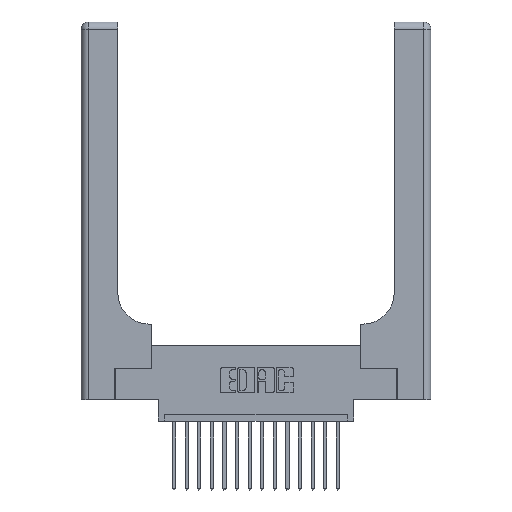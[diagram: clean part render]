
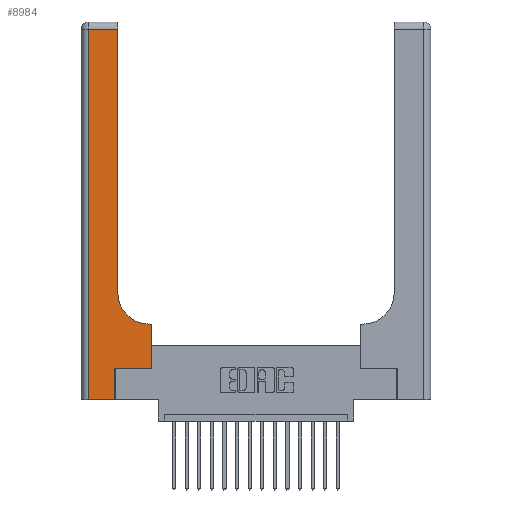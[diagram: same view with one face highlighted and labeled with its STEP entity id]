
A CAD part, top view. The second image highlights one B-rep face of the part: STEP entity #8984.
In plain terms, the highlighted planar face has unit normal (0, 0, 1).
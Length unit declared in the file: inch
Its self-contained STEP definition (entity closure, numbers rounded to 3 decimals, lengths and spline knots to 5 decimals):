
#375 = DIRECTION ( 'NONE',  ( 1., 0., 0. ) ) ;
#637 = ORIENTED_EDGE ( 'NONE', *, *, #4105, .T. ) ;
#830 = VECTOR ( 'NONE', #7267, 39.37008 ) ;
#835 = VERTEX_POINT ( 'NONE', #8999 ) ;
#1026 = CARTESIAN_POINT ( 'NONE',  ( 0.269, 0., 0.37 ) ) ;
#1332 = VERTEX_POINT ( 'NONE', #9746 ) ;
#1426 = LINE ( 'NONE', #15340, #8727 ) ;
#1843 = EDGE_CURVE ( 'NONE', #1332, #18634, #16734, .T. ) ;
#2083 = ORIENTED_EDGE ( 'NONE', *, *, #11551, .T. ) ;
#2517 = VECTOR ( 'NONE', #18983, 39.37008 ) ;
#3129 = DIRECTION ( 'NONE',  ( -1., 0., 0. ) ) ;
#3688 = LINE ( 'NONE', #12869, #2517 ) ;
#4105 = EDGE_CURVE ( 'NONE', #4329, #1332, #11870, .T. ) ;
#4235 = AXIS2_PLACEMENT_3D ( 'NONE', #13280, #10344, #4338 ) ;
#4329 = VERTEX_POINT ( 'NONE', #12420 ) ;
#4338 = DIRECTION ( 'NONE',  ( -1., 0., 0. ) ) ;
#4738 = DIRECTION ( 'NONE',  ( 1., 0., 0. ) ) ;
#4770 = CARTESIAN_POINT ( 'NONE',  ( 0., 2.94, 0.37 ) ) ;
#4840 = CARTESIAN_POINT ( 'NONE',  ( 0.06, 2.94, 0.37 ) ) ;
#6037 = AXIS2_PLACEMENT_3D ( 'NONE', #10881, #18533, #375 ) ;
#6086 = ORIENTED_EDGE ( 'NONE', *, *, #12809, .T. ) ;
#6097 = EDGE_CURVE ( 'NONE', #14502, #4329, #3688, .T. ) ;
#6288 = DIRECTION ( 'NONE',  ( 0., 1., 0. ) ) ;
#6469 = EDGE_LOOP ( 'NONE', ( #2083, #17138, #8055, #637, #8844, #6630, #14395, #15891, #6086 ) ) ;
#6630 = ORIENTED_EDGE ( 'NONE', *, *, #7451, .T. ) ;
#7267 = DIRECTION ( 'NONE',  ( -1., 0., 0. ) ) ;
#7451 = EDGE_CURVE ( 'NONE', #18634, #835, #7834, .T. ) ;
#7834 = LINE ( 'NONE', #14635, #14310 ) ;
#8055 = ORIENTED_EDGE ( 'NONE', *, *, #6097, .T. ) ;
#8470 = CARTESIAN_POINT ( 'NONE',  ( 0.5585, 0.6, 0.37 ) ) ;
#8727 = VECTOR ( 'NONE', #10784, 39.37008 ) ;
#8844 = ORIENTED_EDGE ( 'NONE', *, *, #1843, .T. ) ;
#8984 = ADVANCED_FACE ( 'NONE', ( #17605 ), #11674, .F. ) ;
#8999 = CARTESIAN_POINT ( 'NONE',  ( 0.5585, 0.25, 0.37 ) ) ;
#9328 = LINE ( 'NONE', #11988, #830 ) ;
#9746 = CARTESIAN_POINT ( 'NONE',  ( 0.269, 0., 0.37 ) ) ;
#9819 = EDGE_CURVE ( 'NONE', #835, #11036, #1426, .T. ) ;
#10344 = DIRECTION ( 'NONE',  ( 0., 0., -1. ) ) ;
#10585 = LINE ( 'NONE', #15235, #12728 ) ;
#10784 = DIRECTION ( 'NONE',  ( 0., 1., 0. ) ) ;
#10881 = CARTESIAN_POINT ( 'NONE',  ( 0.5415, 0.85, 0.37 ) ) ;
#11036 = VERTEX_POINT ( 'NONE', #8470 ) ;
#11212 = VERTEX_POINT ( 'NONE', #19307 ) ;
#11500 = CARTESIAN_POINT ( 'NONE',  ( 0.5415, 0.6, 0.37 ) ) ;
#11551 = EDGE_CURVE ( 'NONE', #11212, #17501, #10585, .T. ) ;
#11674 = PLANE ( 'NONE',  #4235 ) ;
#11870 = LINE ( 'NONE', #18333, #14059 ) ;
#11951 = VECTOR ( 'NONE', #19250, 39.37008 ) ;
#11988 = CARTESIAN_POINT ( 'NONE',  ( 0.2915, 0.6, 0.37 ) ) ;
#12420 = CARTESIAN_POINT ( 'NONE',  ( 0.06, 0., 0.37 ) ) ;
#12583 = EDGE_CURVE ( 'NONE', #11036, #14872, #9328, .T. ) ;
#12661 = LINE ( 'NONE', #4770, #15073 ) ;
#12728 = VECTOR ( 'NONE', #6288, 39.37008 ) ;
#12809 = EDGE_CURVE ( 'NONE', #14872, #11212, #14867, .T. ) ;
#12869 = CARTESIAN_POINT ( 'NONE',  ( 0.06, 3., 0.37 ) ) ;
#13280 = CARTESIAN_POINT ( 'NONE',  ( 0., 3., 0.37 ) ) ;
#14059 = VECTOR ( 'NONE', #4738, 39.37008 ) ;
#14068 = CARTESIAN_POINT ( 'NONE',  ( 0.2915, 2.94, 0.37 ) ) ;
#14075 = CARTESIAN_POINT ( 'NONE',  ( 0.269, 0.25, 0.37 ) ) ;
#14310 = VECTOR ( 'NONE', #19046, 39.37008 ) ;
#14395 = ORIENTED_EDGE ( 'NONE', *, *, #9819, .T. ) ;
#14502 = VERTEX_POINT ( 'NONE', #4840 ) ;
#14635 = CARTESIAN_POINT ( 'NONE',  ( 0.269, 0.25, 0.37 ) ) ;
#14867 = CIRCLE ( 'NONE', #6037, 0.25 ) ;
#14872 = VERTEX_POINT ( 'NONE', #11500 ) ;
#15073 = VECTOR ( 'NONE', #3129, 39.37008 ) ;
#15235 = CARTESIAN_POINT ( 'NONE',  ( 0.2915, 3., 0.37 ) ) ;
#15340 = CARTESIAN_POINT ( 'NONE',  ( 0.5585, 0.25, 0.37 ) ) ;
#15891 = ORIENTED_EDGE ( 'NONE', *, *, #12583, .T. ) ;
#16734 = LINE ( 'NONE', #1026, #11951 ) ;
#17138 = ORIENTED_EDGE ( 'NONE', *, *, #17391, .T. ) ;
#17391 = EDGE_CURVE ( 'NONE', #17501, #14502, #12661, .T. ) ;
#17501 = VERTEX_POINT ( 'NONE', #14068 ) ;
#17605 = FACE_OUTER_BOUND ( 'NONE', #6469, .T. ) ;
#18333 = CARTESIAN_POINT ( 'NONE',  ( 0., 0., 0.37 ) ) ;
#18533 = DIRECTION ( 'NONE',  ( 0., 0., -1. ) ) ;
#18634 = VERTEX_POINT ( 'NONE', #14075 ) ;
#18983 = DIRECTION ( 'NONE',  ( 0., -1., 0. ) ) ;
#19046 = DIRECTION ( 'NONE',  ( 1., 0., 0. ) ) ;
#19250 = DIRECTION ( 'NONE',  ( 0., 1., 0. ) ) ;
#19307 = CARTESIAN_POINT ( 'NONE',  ( 0.2915, 0.85, 0.37 ) ) ;
